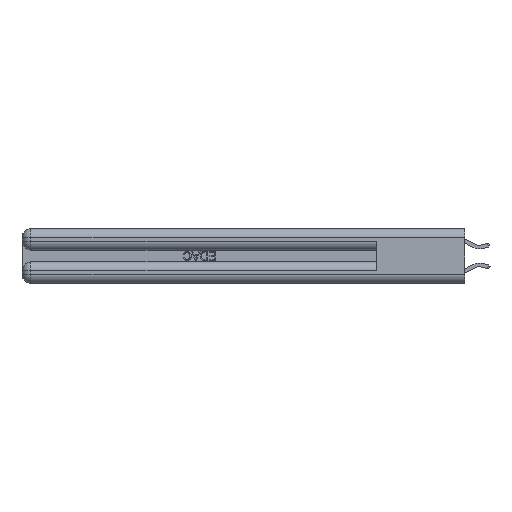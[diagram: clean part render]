
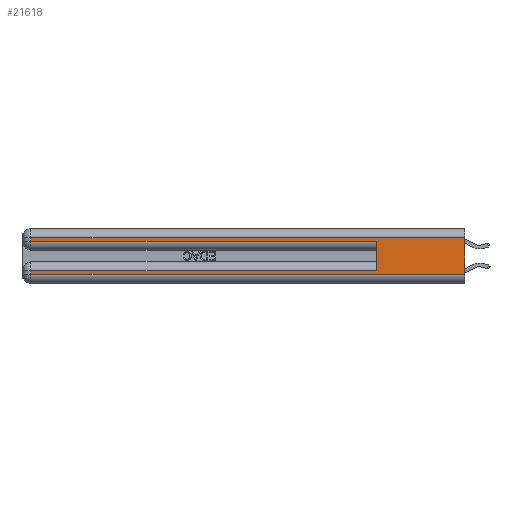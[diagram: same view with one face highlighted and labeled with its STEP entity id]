
A CAD part, left-side view. The second image highlights one B-rep face of the part: STEP entity #21618.
In plain terms, the highlighted planar face has unit normal (-1, 0, 0).
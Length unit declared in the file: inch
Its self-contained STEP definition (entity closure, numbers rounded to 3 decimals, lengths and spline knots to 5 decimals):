
#297 = CARTESIAN_POINT ( 'NONE',  ( 0., 0., 0.37 ) ) ;
#676 = ORIENTED_EDGE ( 'NONE', *, *, #10246, .T. ) ;
#990 = LINE ( 'NONE', #6282, #18655 ) ;
#1159 = EDGE_CURVE ( 'NONE', #18117, #25630, #30223, .T. ) ;
#1433 = ORIENTED_EDGE ( 'NONE', *, *, #24158, .F. ) ;
#1649 = PLANE ( 'NONE',  #9435 ) ;
#2214 = FACE_OUTER_BOUND ( 'NONE', #34729, .T. ) ;
#2550 = ORIENTED_EDGE ( 'NONE', *, *, #16631, .T. ) ;
#2912 = VECTOR ( 'NONE', #9283, 39.37008 ) ;
#3464 = EDGE_CURVE ( 'NONE', #12676, #25006, #30088, .T. ) ;
#3479 = ORIENTED_EDGE ( 'NONE', *, *, #35727, .F. ) ;
#3698 = VECTOR ( 'NONE', #5594, 39.37008 ) ;
#3715 = DIRECTION ( 'NONE',  ( 0., -1., 0. ) ) ;
#4129 = DIRECTION ( 'NONE',  ( 0., 1., 0. ) ) ;
#5353 = LINE ( 'NONE', #22795, #6856 ) ;
#5491 = CARTESIAN_POINT ( 'NONE',  ( 0., 2.94, 0.31 ) ) ;
#5594 = DIRECTION ( 'NONE',  ( 0., 0., -1. ) ) ;
#5806 = CARTESIAN_POINT ( 'NONE',  ( 0., 0., 0.285 ) ) ;
#6282 = CARTESIAN_POINT ( 'NONE',  ( 0., 2.94, 0.37 ) ) ;
#6856 = VECTOR ( 'NONE', #13857, 39.37008 ) ;
#7053 = VECTOR ( 'NONE', #3715, 39.37008 ) ;
#8863 = VECTOR ( 'NONE', #19352, 39.37008 ) ;
#9283 = DIRECTION ( 'NONE',  ( 0., -1., 0. ) ) ;
#9435 = AXIS2_PLACEMENT_3D ( 'NONE', #13740, #25335, #22481 ) ;
#9484 = VERTEX_POINT ( 'NONE', #12303 ) ;
#9745 = CARTESIAN_POINT ( 'NONE',  ( 0., 2.94, 0.37 ) ) ;
#10246 = EDGE_CURVE ( 'NONE', #25630, #9484, #26475, .T. ) ;
#11072 = CARTESIAN_POINT ( 'NONE',  ( 0., 2.94, 0.085 ) ) ;
#12105 = CARTESIAN_POINT ( 'NONE',  ( 0., 0., 0.06 ) ) ;
#12303 = CARTESIAN_POINT ( 'NONE',  ( 0., 0.6, 0.285 ) ) ;
#12341 = ORIENTED_EDGE ( 'NONE', *, *, #24038, .T. ) ;
#12676 = VERTEX_POINT ( 'NONE', #13632 ) ;
#13632 = CARTESIAN_POINT ( 'NONE',  ( 0., 0.6, 0.085 ) ) ;
#13740 = CARTESIAN_POINT ( 'NONE',  ( 0., 0., 0.37 ) ) ;
#13857 = DIRECTION ( 'NONE',  ( 0., 1., 0. ) ) ;
#15430 = ORIENTED_EDGE ( 'NONE', *, *, #3464, .T. ) ;
#16631 = EDGE_CURVE ( 'NONE', #22440, #18117, #5353, .T. ) ;
#16969 = LINE ( 'NONE', #297, #3698 ) ;
#18117 = VERTEX_POINT ( 'NONE', #5491 ) ;
#18655 = VECTOR ( 'NONE', #32808, 39.37008 ) ;
#19352 = DIRECTION ( 'NONE',  ( 0., 0., -1. ) ) ;
#19368 = ORIENTED_EDGE ( 'NONE', *, *, #1159, .T. ) ;
#20948 = VECTOR ( 'NONE', #4129, 39.37008 ) ;
#21600 = CARTESIAN_POINT ( 'NONE',  ( 0., 2.94, 0.06 ) ) ;
#21618 = ADVANCED_FACE ( 'NONE', ( #2214 ), #1649, .F. ) ;
#21636 = DIRECTION ( 'NONE',  ( 0., 0., 1. ) ) ;
#22440 = VERTEX_POINT ( 'NONE', #31690 ) ;
#22481 = DIRECTION ( 'NONE',  ( 0., 0., -1. ) ) ;
#22795 = CARTESIAN_POINT ( 'NONE',  ( 0., 0., 0.31 ) ) ;
#23315 = VECTOR ( 'NONE', #21636, 39.37008 ) ;
#24038 = EDGE_CURVE ( 'NONE', #25006, #36322, #990, .T. ) ;
#24158 = EDGE_CURVE ( 'NONE', #12676, #9484, #30346, .T. ) ;
#25006 = VERTEX_POINT ( 'NONE', #11072 ) ;
#25335 = DIRECTION ( 'NONE',  ( 1., 0., 0. ) ) ;
#25630 = VERTEX_POINT ( 'NONE', #29751 ) ;
#25648 = EDGE_CURVE ( 'NONE', #36322, #34795, #37206, .T. ) ;
#26475 = LINE ( 'NONE', #5806, #7053 ) ;
#29076 = ORIENTED_EDGE ( 'NONE', *, *, #25648, .T. ) ;
#29751 = CARTESIAN_POINT ( 'NONE',  ( 0., 2.94, 0.285 ) ) ;
#30088 = LINE ( 'NONE', #35770, #20948 ) ;
#30223 = LINE ( 'NONE', #9745, #8863 ) ;
#30346 = LINE ( 'NONE', #36575, #23315 ) ;
#31690 = CARTESIAN_POINT ( 'NONE',  ( 0., 0., 0.31 ) ) ;
#32808 = DIRECTION ( 'NONE',  ( 0., 0., -1. ) ) ;
#34306 = CARTESIAN_POINT ( 'NONE',  ( 0., 0., 0.06 ) ) ;
#34729 = EDGE_LOOP ( 'NONE', ( #3479, #2550, #19368, #676, #1433, #15430, #12341, #29076 ) ) ;
#34795 = VERTEX_POINT ( 'NONE', #34306 ) ;
#35727 = EDGE_CURVE ( 'NONE', #22440, #34795, #16969, .T. ) ;
#35770 = CARTESIAN_POINT ( 'NONE',  ( 0., 0., 0.085 ) ) ;
#36322 = VERTEX_POINT ( 'NONE', #21600 ) ;
#36575 = CARTESIAN_POINT ( 'NONE',  ( 0., 0.6, 0.145 ) ) ;
#37206 = LINE ( 'NONE', #12105, #2912 ) ;
